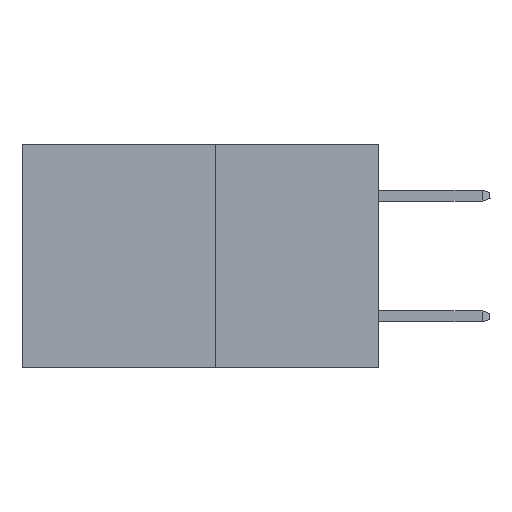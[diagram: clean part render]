
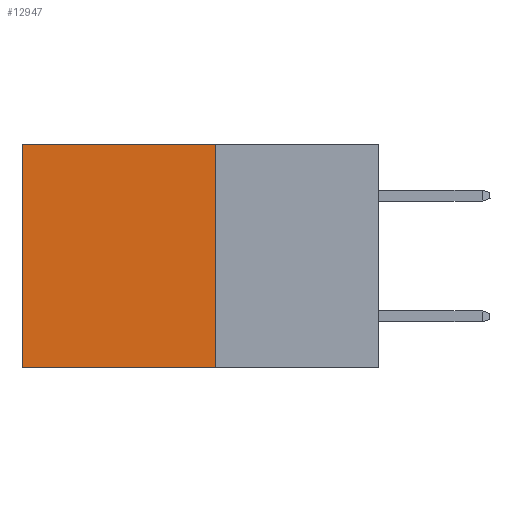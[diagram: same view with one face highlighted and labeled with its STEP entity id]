
A CAD part, left-side view. The second image highlights one B-rep face of the part: STEP entity #12947.
In plain terms, the highlighted planar face has unit normal (-1, 0, 0).
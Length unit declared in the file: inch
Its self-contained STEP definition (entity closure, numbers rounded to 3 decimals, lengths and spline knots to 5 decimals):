
#67 = CARTESIAN_POINT ( 'NONE',  ( 0.277, 0.59, -0.37 ) ) ;
#715 = DIRECTION ( 'NONE',  ( 0., 0., -1. ) ) ;
#794 = VECTOR ( 'NONE', #10818, 39.37008 ) ;
#1099 = VECTOR ( 'NONE', #10022, 39.37008 ) ;
#2409 = EDGE_CURVE ( 'NONE', #4152, #4641, #6360, .T. ) ;
#2664 = FACE_OUTER_BOUND ( 'NONE', #7393, .T. ) ;
#3255 = ORIENTED_EDGE ( 'NONE', *, *, #14289, .T. ) ;
#3770 = ORIENTED_EDGE ( 'NONE', *, *, #11910, .F. ) ;
#4152 = VERTEX_POINT ( 'NONE', #12507 ) ;
#4479 = LINE ( 'NONE', #67, #14078 ) ;
#4494 = CARTESIAN_POINT ( 'NONE',  ( 0.277, 0.27, -0.37 ) ) ;
#4641 = VERTEX_POINT ( 'NONE', #11608 ) ;
#4760 = ORIENTED_EDGE ( 'NONE', *, *, #12588, .T. ) ;
#4943 = CARTESIAN_POINT ( 'NONE',  ( 0.277, 0.27, 0. ) ) ;
#5121 = LINE ( 'NONE', #7671, #14670 ) ;
#5301 = LINE ( 'NONE', #4943, #1099 ) ;
#6360 = LINE ( 'NONE', #10055, #794 ) ;
#6726 = ORIENTED_EDGE ( 'NONE', *, *, #2409, .F. ) ;
#7239 = CARTESIAN_POINT ( 'NONE',  ( 0.277, 0.27, 0. ) ) ;
#7393 = EDGE_LOOP ( 'NONE', ( #4760, #6726, #3770, #3255 ) ) ;
#7671 = CARTESIAN_POINT ( 'NONE',  ( 0.277, 0.27, -0.37 ) ) ;
#8287 = CARTESIAN_POINT ( 'NONE',  ( 0.277, 0.59, 0. ) ) ;
#8317 = DIRECTION ( 'NONE',  ( 1., 0., 0. ) ) ;
#8984 = DIRECTION ( 'NONE',  ( 0., 0., -1. ) ) ;
#9627 = AXIS2_PLACEMENT_3D ( 'NONE', #4494, #8317, #715 ) ;
#10022 = DIRECTION ( 'NONE',  ( 0., 1., 0. ) ) ;
#10055 = CARTESIAN_POINT ( 'NONE',  ( 0.277, 0.27, -0.37 ) ) ;
#10818 = DIRECTION ( 'NONE',  ( 0., 1., 0. ) ) ;
#11608 = CARTESIAN_POINT ( 'NONE',  ( 0.277, 0.59, -0.37 ) ) ;
#11910 = EDGE_CURVE ( 'NONE', #13058, #4152, #5121, .T. ) ;
#12507 = CARTESIAN_POINT ( 'NONE',  ( 0.277, 0.27, -0.37 ) ) ;
#12588 = EDGE_CURVE ( 'NONE', #14721, #4641, #4479, .T. ) ;
#12947 = ADVANCED_FACE ( 'NONE', ( #2664 ), #15709, .F. ) ;
#13058 = VERTEX_POINT ( 'NONE', #7239 ) ;
#14078 = VECTOR ( 'NONE', #8984, 39.37008 ) ;
#14289 = EDGE_CURVE ( 'NONE', #13058, #14721, #5301, .T. ) ;
#14670 = VECTOR ( 'NONE', #15082, 39.37008 ) ;
#14721 = VERTEX_POINT ( 'NONE', #8287 ) ;
#15082 = DIRECTION ( 'NONE',  ( 0., 0., -1. ) ) ;
#15709 = PLANE ( 'NONE',  #9627 ) ;
